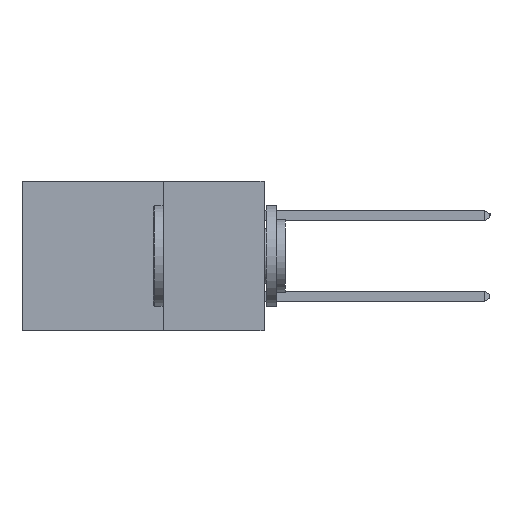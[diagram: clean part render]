
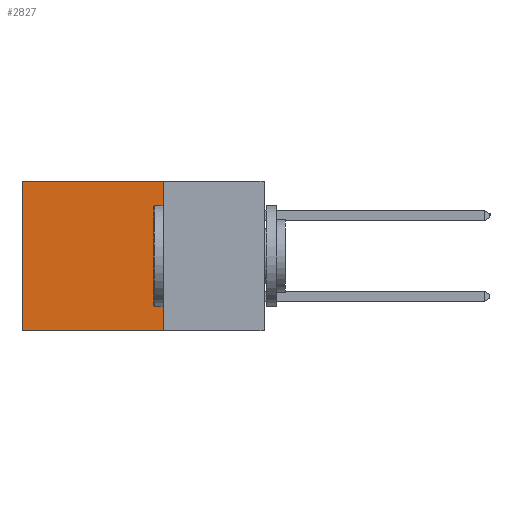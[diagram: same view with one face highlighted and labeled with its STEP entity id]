
A CAD part, left-side view. The second image highlights one B-rep face of the part: STEP entity #2827.
In plain terms, the highlighted planar face has unit normal (-1, 0, 0).
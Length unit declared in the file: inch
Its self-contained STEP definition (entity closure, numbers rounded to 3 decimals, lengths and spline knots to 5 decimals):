
#250 = AXIS2_PLACEMENT_3D ( 'NONE', #4788, #10207, #4701 ) ;
#281 = DIRECTION ( 'NONE',  ( 0., 1., 0. ) ) ;
#838 = EDGE_CURVE ( 'NONE', #16587, #14342, #16328, .T. ) ;
#975 = CARTESIAN_POINT ( 'NONE',  ( 0.2615, 0.6, -0.37 ) ) ;
#1044 = EDGE_CURVE ( 'NONE', #16587, #2249, #9820, .T. ) ;
#2249 = VERTEX_POINT ( 'NONE', #10697 ) ;
#2827 = ADVANCED_FACE ( 'NONE', ( #7558 ), #14252, .F. ) ;
#3730 = LINE ( 'NONE', #13280, #16921 ) ;
#4658 = CARTESIAN_POINT ( 'NONE',  ( 0.2615, 0.25, -0.37 ) ) ;
#4701 = DIRECTION ( 'NONE',  ( 0., 0., -1. ) ) ;
#4788 = CARTESIAN_POINT ( 'NONE',  ( 0.2615, 0.25, -0.37 ) ) ;
#5598 = ORIENTED_EDGE ( 'NONE', *, *, #14566, .F. ) ;
#5636 = CARTESIAN_POINT ( 'NONE',  ( 0.2615, 0.25, 0. ) ) ;
#6098 = CARTESIAN_POINT ( 'NONE',  ( 0.2615, 0.25, 0. ) ) ;
#6755 = VECTOR ( 'NONE', #15103, 39.37008 ) ;
#7137 = ORIENTED_EDGE ( 'NONE', *, *, #1044, .F. ) ;
#7558 = FACE_OUTER_BOUND ( 'NONE', #9121, .T. ) ;
#8379 = EDGE_CURVE ( 'NONE', #14342, #11215, #3730, .T. ) ;
#8581 = VECTOR ( 'NONE', #281, 39.37008 ) ;
#8659 = ORIENTED_EDGE ( 'NONE', *, *, #838, .T. ) ;
#9121 = EDGE_LOOP ( 'NONE', ( #13362, #5598, #7137, #8659 ) ) ;
#9820 = LINE ( 'NONE', #4658, #10211 ) ;
#10207 = DIRECTION ( 'NONE',  ( 1., 0., 0. ) ) ;
#10211 = VECTOR ( 'NONE', #13853, 39.37008 ) ;
#10565 = DIRECTION ( 'NONE',  ( 0., 0., -1. ) ) ;
#10697 = CARTESIAN_POINT ( 'NONE',  ( 0.2615, 0.25, -0.37 ) ) ;
#11096 = CARTESIAN_POINT ( 'NONE',  ( 0.2615, 0.6, 0. ) ) ;
#11215 = VERTEX_POINT ( 'NONE', #975 ) ;
#12226 = CARTESIAN_POINT ( 'NONE',  ( 0.2615, 0.25, -0.37 ) ) ;
#13280 = CARTESIAN_POINT ( 'NONE',  ( 0.2615, 0.6, -0.37 ) ) ;
#13362 = ORIENTED_EDGE ( 'NONE', *, *, #8379, .T. ) ;
#13853 = DIRECTION ( 'NONE',  ( 0., 0., -1. ) ) ;
#14252 = PLANE ( 'NONE',  #250 ) ;
#14342 = VERTEX_POINT ( 'NONE', #11096 ) ;
#14566 = EDGE_CURVE ( 'NONE', #2249, #11215, #15205, .T. ) ;
#15103 = DIRECTION ( 'NONE',  ( 0., 1., 0. ) ) ;
#15205 = LINE ( 'NONE', #12226, #8581 ) ;
#16328 = LINE ( 'NONE', #5636, #6755 ) ;
#16587 = VERTEX_POINT ( 'NONE', #6098 ) ;
#16921 = VECTOR ( 'NONE', #10565, 39.37008 ) ;
